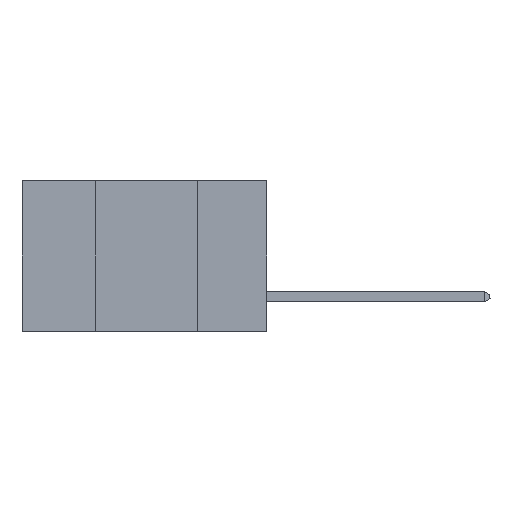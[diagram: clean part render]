
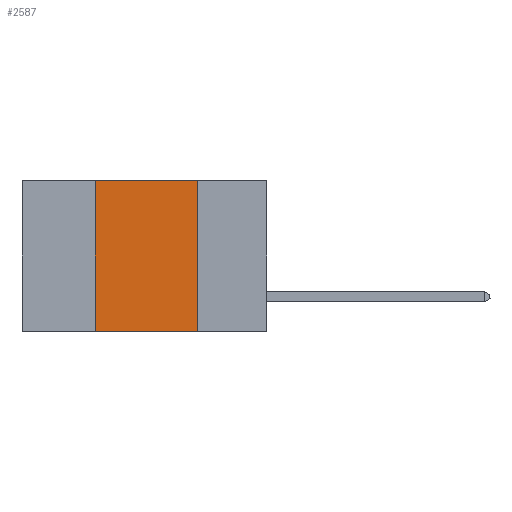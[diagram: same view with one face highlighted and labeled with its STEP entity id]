
A CAD part, left-side view. The second image highlights one B-rep face of the part: STEP entity #2587.
In plain terms, the highlighted planar face has unit normal (-1, 0, 0).
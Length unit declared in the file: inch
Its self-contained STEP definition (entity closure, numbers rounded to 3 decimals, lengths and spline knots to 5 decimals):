
#271 = ORIENTED_EDGE ( 'NONE', *, *, #10049, .F. ) ;
#595 = CARTESIAN_POINT ( 'NONE',  ( 0., 0.42, 0. ) ) ;
#713 = CARTESIAN_POINT ( 'NONE',  ( 0., 0.17, 0. ) ) ;
#854 = LINE ( 'NONE', #2992, #9680 ) ;
#1340 = VERTEX_POINT ( 'NONE', #1968 ) ;
#1624 = ORIENTED_EDGE ( 'NONE', *, *, #10378, .F. ) ;
#1968 = CARTESIAN_POINT ( 'NONE',  ( 0., 0.17, -0.37 ) ) ;
#2086 = VECTOR ( 'NONE', #2643, 39.37008 ) ;
#2179 = DIRECTION ( 'NONE',  ( 1., 0., 0. ) ) ;
#2273 = ORIENTED_EDGE ( 'NONE', *, *, #5249, .T. ) ;
#2381 = DIRECTION ( 'NONE',  ( 0., 0., -1. ) ) ;
#2587 = ADVANCED_FACE ( 'NONE', ( #10632 ), #7480, .F. ) ;
#2643 = DIRECTION ( 'NONE',  ( 0., 0., 1. ) ) ;
#2777 = AXIS2_PLACEMENT_3D ( 'NONE', #8256, #2179, #2381 ) ;
#2894 = ORIENTED_EDGE ( 'NONE', *, *, #8706, .F. ) ;
#2992 = CARTESIAN_POINT ( 'NONE',  ( 0., 0.6, 0. ) ) ;
#3506 = VECTOR ( 'NONE', #9754, 39.37008 ) ;
#4027 = CARTESIAN_POINT ( 'NONE',  ( 0., 0.42, -0.37 ) ) ;
#4751 = DIRECTION ( 'NONE',  ( 0., -1., 0. ) ) ;
#5249 = EDGE_CURVE ( 'NONE', #5623, #1340, #5317, .T. ) ;
#5317 = LINE ( 'NONE', #8803, #8199 ) ;
#5623 = VERTEX_POINT ( 'NONE', #4027 ) ;
#5677 = DIRECTION ( 'NONE',  ( 0., -1., 0. ) ) ;
#5732 = LINE ( 'NONE', #713, #3506 ) ;
#6034 = VERTEX_POINT ( 'NONE', #595 ) ;
#6906 = LINE ( 'NONE', #10087, #2086 ) ;
#7209 = EDGE_LOOP ( 'NONE', ( #1624, #2894, #271, #2273 ) ) ;
#7480 = PLANE ( 'NONE',  #2777 ) ;
#8141 = VERTEX_POINT ( 'NONE', #8947 ) ;
#8199 = VECTOR ( 'NONE', #4751, 39.37008 ) ;
#8256 = CARTESIAN_POINT ( 'NONE',  ( 0., 0.6, 0. ) ) ;
#8706 = EDGE_CURVE ( 'NONE', #6034, #8141, #854, .T. ) ;
#8803 = CARTESIAN_POINT ( 'NONE',  ( 0., 0.6, -0.37 ) ) ;
#8947 = CARTESIAN_POINT ( 'NONE',  ( 0., 0.17, 0. ) ) ;
#9680 = VECTOR ( 'NONE', #5677, 39.37008 ) ;
#9754 = DIRECTION ( 'NONE',  ( 0., 0., -1. ) ) ;
#10049 = EDGE_CURVE ( 'NONE', #5623, #6034, #6906, .T. ) ;
#10087 = CARTESIAN_POINT ( 'NONE',  ( 0., 0.42, 0. ) ) ;
#10378 = EDGE_CURVE ( 'NONE', #8141, #1340, #5732, .T. ) ;
#10632 = FACE_OUTER_BOUND ( 'NONE', #7209, .T. ) ;
